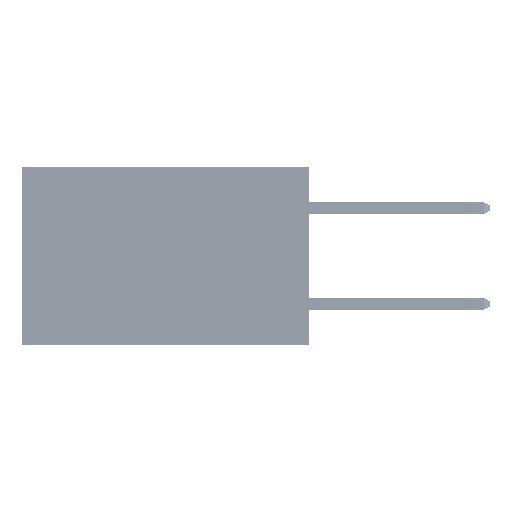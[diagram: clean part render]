
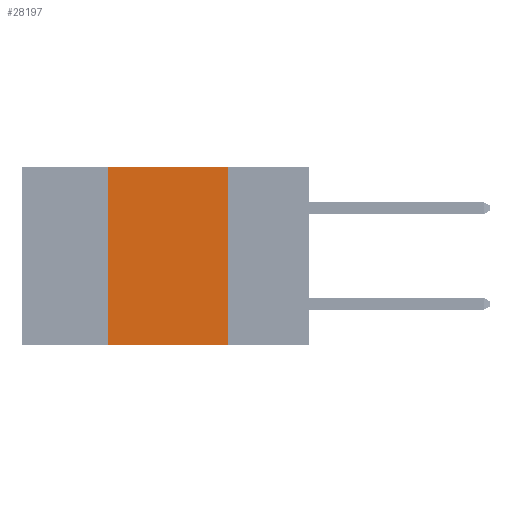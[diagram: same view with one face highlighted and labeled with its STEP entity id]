
A CAD part, left-side view. The second image highlights one B-rep face of the part: STEP entity #28197.
In plain terms, the highlighted planar face has unit normal (-1, 0, 0).
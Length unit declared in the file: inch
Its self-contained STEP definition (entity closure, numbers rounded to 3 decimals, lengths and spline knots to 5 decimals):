
#1016 = VECTOR ( 'NONE', #40102, 39.37008 ) ;
#2241 = LINE ( 'NONE', #20936, #1016 ) ;
#4501 = DIRECTION ( 'NONE',  ( 0., 0., -1. ) ) ;
#5578 = ORIENTED_EDGE ( 'NONE', *, *, #17473, .F. ) ;
#6789 = CARTESIAN_POINT ( 'NONE',  ( 0., 0.17, 0. ) ) ;
#6860 = DIRECTION ( 'NONE',  ( 0., -1., 0. ) ) ;
#7445 = ORIENTED_EDGE ( 'NONE', *, *, #35204, .F. ) ;
#9474 = DIRECTION ( 'NONE',  ( 0., 0., 1. ) ) ;
#10845 = AXIS2_PLACEMENT_3D ( 'NONE', #29267, #13922, #17490 ) ;
#11924 = LINE ( 'NONE', #28090, #41490 ) ;
#12822 = EDGE_CURVE ( 'NONE', #26213, #48734, #2241, .T. ) ;
#13922 = DIRECTION ( 'NONE',  ( 1., 0., 0. ) ) ;
#15616 = CARTESIAN_POINT ( 'NONE',  ( 0., 0.42, -0.37 ) ) ;
#17473 = EDGE_CURVE ( 'NONE', #48734, #29776, #44728, .T. ) ;
#17490 = DIRECTION ( 'NONE',  ( 0., 0., -1. ) ) ;
#18848 = FACE_OUTER_BOUND ( 'NONE', #28674, .T. ) ;
#19078 = CARTESIAN_POINT ( 'NONE',  ( 0., 0.6, -0.37 ) ) ;
#20598 = VECTOR ( 'NONE', #4501, 39.37008 ) ;
#20936 = CARTESIAN_POINT ( 'NONE',  ( 0., 0.6, 0. ) ) ;
#25235 = PLANE ( 'NONE',  #10845 ) ;
#26213 = VERTEX_POINT ( 'NONE', #46208 ) ;
#28090 = CARTESIAN_POINT ( 'NONE',  ( 0., 0.42, 0. ) ) ;
#28197 = ADVANCED_FACE ( 'NONE', ( #18848 ), #25235, .F. ) ;
#28674 = EDGE_LOOP ( 'NONE', ( #5578, #31435, #7445, #41902 ) ) ;
#29267 = CARTESIAN_POINT ( 'NONE',  ( 0., 0.6, 0. ) ) ;
#29776 = VERTEX_POINT ( 'NONE', #42626 ) ;
#31156 = VERTEX_POINT ( 'NONE', #15616 ) ;
#31435 = ORIENTED_EDGE ( 'NONE', *, *, #12822, .F. ) ;
#31723 = CARTESIAN_POINT ( 'NONE',  ( 0., 0.17, 0. ) ) ;
#35204 = EDGE_CURVE ( 'NONE', #31156, #26213, #11924, .T. ) ;
#37371 = EDGE_CURVE ( 'NONE', #31156, #29776, #39172, .T. ) ;
#39172 = LINE ( 'NONE', #19078, #45245 ) ;
#40102 = DIRECTION ( 'NONE',  ( 0., -1., 0. ) ) ;
#41490 = VECTOR ( 'NONE', #9474, 39.37008 ) ;
#41902 = ORIENTED_EDGE ( 'NONE', *, *, #37371, .T. ) ;
#42626 = CARTESIAN_POINT ( 'NONE',  ( 0., 0.17, -0.37 ) ) ;
#44728 = LINE ( 'NONE', #31723, #20598 ) ;
#45245 = VECTOR ( 'NONE', #6860, 39.37008 ) ;
#46208 = CARTESIAN_POINT ( 'NONE',  ( 0., 0.42, 0. ) ) ;
#48734 = VERTEX_POINT ( 'NONE', #6789 ) ;
